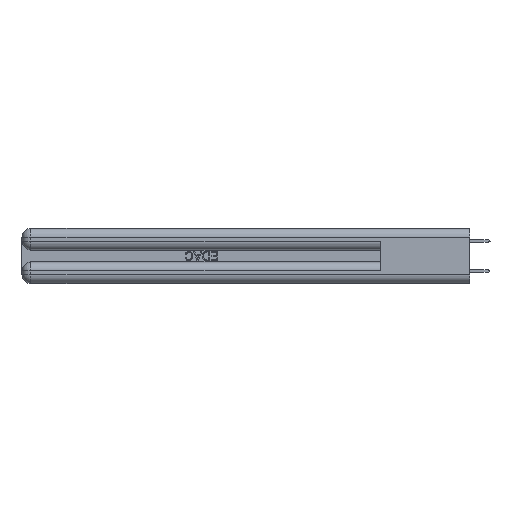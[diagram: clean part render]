
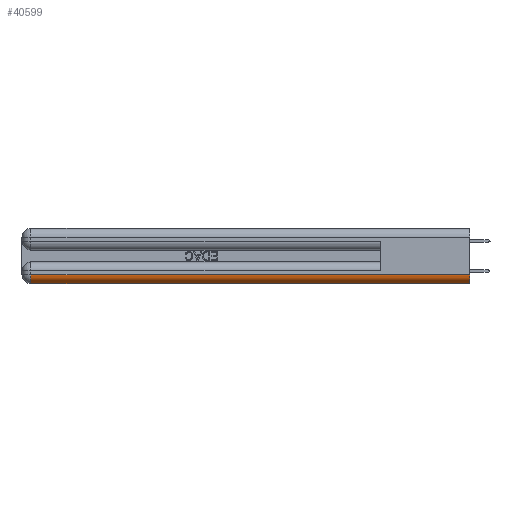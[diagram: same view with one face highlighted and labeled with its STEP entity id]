
A CAD part, left-side view. The second image highlights one B-rep face of the part: STEP entity #40599.
In plain terms, the highlighted cylindrical face has radius 1.524 mm (diameter 3.048 mm), a partial arc.
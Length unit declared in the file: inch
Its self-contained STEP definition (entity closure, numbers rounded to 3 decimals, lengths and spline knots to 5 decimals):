
#328 = AXIS2_PLACEMENT_3D ( 'NONE', #13449, #2167, #29077 ) ;
#2167 = DIRECTION ( 'NONE',  ( 0., 1., 0. ) ) ;
#2836 = LINE ( 'NONE', #17413, #39654 ) ;
#7622 = CARTESIAN_POINT ( 'NONE',  ( 0.06, 0., 0.06 ) ) ;
#9836 = EDGE_CURVE ( 'NONE', #30443, #40415, #2836, .T. ) ;
#9859 = ORIENTED_EDGE ( 'NONE', *, *, #47041, .F. ) ;
#12327 = ORIENTED_EDGE ( 'NONE', *, *, #9836, .F. ) ;
#13118 = CARTESIAN_POINT ( 'NONE',  ( 0.06, 2.94, 0. ) ) ;
#13449 = CARTESIAN_POINT ( 'NONE',  ( 0.06, 2.94, 0.06 ) ) ;
#15483 = AXIS2_PLACEMENT_3D ( 'NONE', #48442, #17955, #25144 ) ;
#17390 = DIRECTION ( 'NONE',  ( 0., 1., 0. ) ) ;
#17413 = CARTESIAN_POINT ( 'NONE',  ( 0., 0., 0.06 ) ) ;
#17955 = DIRECTION ( 'NONE',  ( 0., 1., 0. ) ) ;
#19080 = CIRCLE ( 'NONE', #328, 0.06 ) ;
#21765 = DIRECTION ( 'NONE',  ( 0., -1., 0. ) ) ;
#24668 = ORIENTED_EDGE ( 'NONE', *, *, #45839, .F. ) ;
#25085 = CARTESIAN_POINT ( 'NONE',  ( 0.06, 3., 0. ) ) ;
#25144 = DIRECTION ( 'NONE',  ( 0., 0., 1. ) ) ;
#29008 = CYLINDRICAL_SURFACE ( 'NONE', #15483, 0.06 ) ;
#29077 = DIRECTION ( 'NONE',  ( 0., 0., 1. ) ) ;
#30117 = CARTESIAN_POINT ( 'NONE',  ( 0.06, 0., 0. ) ) ;
#30443 = VERTEX_POINT ( 'NONE', #42126 ) ;
#33331 = FACE_OUTER_BOUND ( 'NONE', #40636, .T. ) ;
#33753 = VECTOR ( 'NONE', #17390, 39.37008 ) ;
#35026 = DIRECTION ( 'NONE',  ( 0., -1., 0. ) ) ;
#36856 = VERTEX_POINT ( 'NONE', #13118 ) ;
#38614 = ORIENTED_EDGE ( 'NONE', *, *, #47862, .F. ) ;
#39654 = VECTOR ( 'NONE', #21765, 39.37008 ) ;
#40415 = VERTEX_POINT ( 'NONE', #46247 ) ;
#40599 = ADVANCED_FACE ( 'NONE', ( #33331 ), #29008, .T. ) ;
#40636 = EDGE_LOOP ( 'NONE', ( #24668, #12327, #38614, #9859 ) ) ;
#42126 = CARTESIAN_POINT ( 'NONE',  ( 0., 2.94, 0.06 ) ) ;
#45811 = LINE ( 'NONE', #25085, #33753 ) ;
#45839 = EDGE_CURVE ( 'NONE', #40415, #50337, #47578, .T. ) ;
#45966 = AXIS2_PLACEMENT_3D ( 'NONE', #7622, #35026, #49897 ) ;
#46247 = CARTESIAN_POINT ( 'NONE',  ( 0., 0., 0.06 ) ) ;
#47041 = EDGE_CURVE ( 'NONE', #50337, #36856, #45811, .T. ) ;
#47578 = CIRCLE ( 'NONE', #45966, 0.06 ) ;
#47862 = EDGE_CURVE ( 'NONE', #36856, #30443, #19080, .T. ) ;
#48442 = CARTESIAN_POINT ( 'NONE',  ( 0.06, 0., 0.06 ) ) ;
#49897 = DIRECTION ( 'NONE',  ( 0., 0., 1. ) ) ;
#50337 = VERTEX_POINT ( 'NONE', #30117 ) ;
